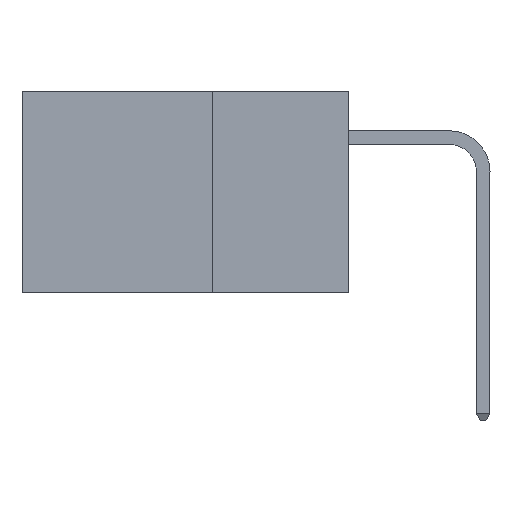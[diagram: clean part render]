
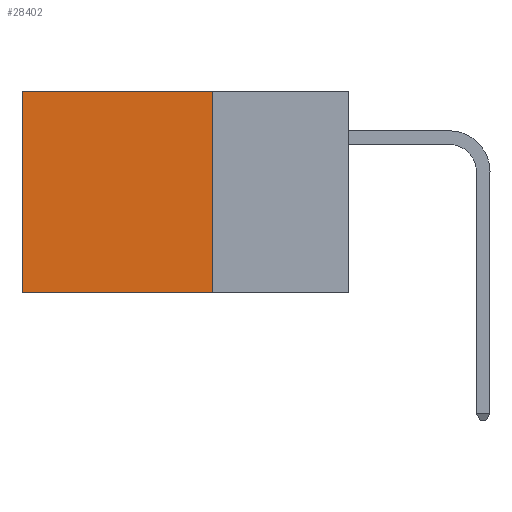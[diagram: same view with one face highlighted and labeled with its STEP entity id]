
A CAD part, left-side view. The second image highlights one B-rep face of the part: STEP entity #28402.
In plain terms, the highlighted planar face has unit normal (-1, 0, 0).
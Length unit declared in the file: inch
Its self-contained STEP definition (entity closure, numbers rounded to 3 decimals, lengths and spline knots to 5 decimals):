
#825 = EDGE_CURVE ( 'NONE', #4889, #2449, #15610, .T. ) ;
#1557 = CARTESIAN_POINT ( 'NONE',  ( 0.2875, 0.25, -0.37 ) ) ;
#2449 = VERTEX_POINT ( 'NONE', #35563 ) ;
#2537 = CARTESIAN_POINT ( 'NONE',  ( 0.2875, 0.6, -0.37 ) ) ;
#2823 = CARTESIAN_POINT ( 'NONE',  ( 0.2875, 0.25, 0. ) ) ;
#3013 = DIRECTION ( 'NONE',  ( 0., 0., -1. ) ) ;
#3148 = VERTEX_POINT ( 'NONE', #1557 ) ;
#4426 = DIRECTION ( 'NONE',  ( 0., 1., 0. ) ) ;
#4721 = DIRECTION ( 'NONE',  ( 0., 1., 0. ) ) ;
#4889 = VERTEX_POINT ( 'NONE', #2823 ) ;
#8122 = ORIENTED_EDGE ( 'NONE', *, *, #825, .T. ) ;
#8167 = PLANE ( 'NONE',  #18198 ) ;
#8294 = DIRECTION ( 'NONE',  ( 1., 0., 0. ) ) ;
#10477 = VERTEX_POINT ( 'NONE', #2537 ) ;
#10720 = VECTOR ( 'NONE', #4721, 39.37008 ) ;
#10774 = FACE_OUTER_BOUND ( 'NONE', #36690, .T. ) ;
#10863 = LINE ( 'NONE', #24974, #10720 ) ;
#13287 = CARTESIAN_POINT ( 'NONE',  ( 0.2875, 0.25, 0. ) ) ;
#13656 = VECTOR ( 'NONE', #3013, 39.37008 ) ;
#13988 = DIRECTION ( 'NONE',  ( 0., 0., -1. ) ) ;
#15547 = VECTOR ( 'NONE', #4426, 39.37008 ) ;
#15610 = LINE ( 'NONE', #13287, #15547 ) ;
#17123 = EDGE_CURVE ( 'NONE', #3148, #10477, #10863, .T. ) ;
#18198 = AXIS2_PLACEMENT_3D ( 'NONE', #36714, #8294, #28443 ) ;
#18816 = ORIENTED_EDGE ( 'NONE', *, *, #31703, .T. ) ;
#19409 = VECTOR ( 'NONE', #13988, 39.37008 ) ;
#23224 = ORIENTED_EDGE ( 'NONE', *, *, #31260, .F. ) ;
#23267 = CARTESIAN_POINT ( 'NONE',  ( 0.2875, 0.25, 0. ) ) ;
#23835 = ORIENTED_EDGE ( 'NONE', *, *, #17123, .F. ) ;
#24974 = CARTESIAN_POINT ( 'NONE',  ( 0.2875, 0.25, -0.37 ) ) ;
#28402 = ADVANCED_FACE ( 'NONE', ( #10774 ), #8167, .F. ) ;
#28443 = DIRECTION ( 'NONE',  ( 0., 0., -1. ) ) ;
#28754 = LINE ( 'NONE', #30965, #19409 ) ;
#30965 = CARTESIAN_POINT ( 'NONE',  ( 0.2875, 0.6, 0. ) ) ;
#31260 = EDGE_CURVE ( 'NONE', #4889, #3148, #36140, .T. ) ;
#31703 = EDGE_CURVE ( 'NONE', #2449, #10477, #28754, .T. ) ;
#35563 = CARTESIAN_POINT ( 'NONE',  ( 0.2875, 0.6, 0. ) ) ;
#36140 = LINE ( 'NONE', #23267, #13656 ) ;
#36690 = EDGE_LOOP ( 'NONE', ( #18816, #23835, #23224, #8122 ) ) ;
#36714 = CARTESIAN_POINT ( 'NONE',  ( 0.2875, 0.25, 0. ) ) ;
